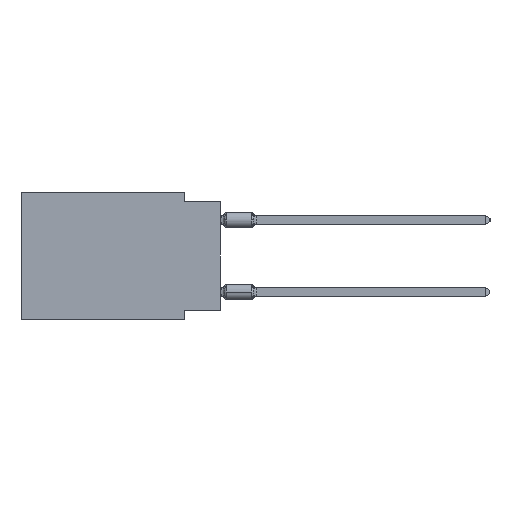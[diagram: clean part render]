
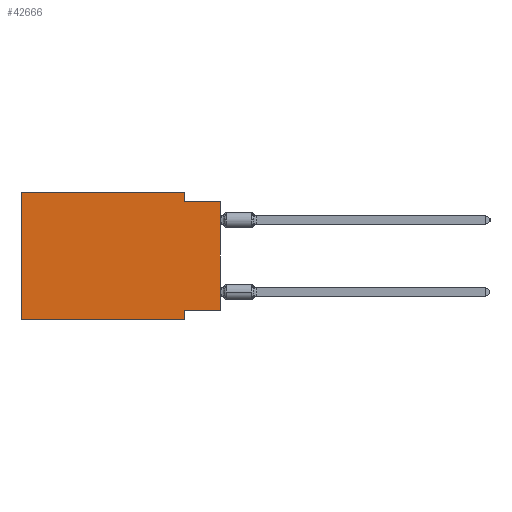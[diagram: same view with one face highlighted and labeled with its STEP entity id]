
A CAD part, left-side view. The second image highlights one B-rep face of the part: STEP entity #42666.
In plain terms, the highlighted planar face has unit normal (-1, 0, 0).
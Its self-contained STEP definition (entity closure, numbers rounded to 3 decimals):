
#12 = DIRECTION ( 'NONE',  ( 0., 0., -1. ) ) ;
#347 = LINE ( 'NONE', #47670, #58235 ) ;
#3822 = ORIENTED_EDGE ( 'NONE', *, *, #8270, .F. ) ;
#6979 = LINE ( 'NONE', #64171, #62223 ) ;
#8270 = EDGE_CURVE ( 'NONE', #39249, #8826, #15601, .T. ) ;
#8386 = DIRECTION ( 'NONE',  ( 0., 0., -1. ) ) ;
#8826 = VERTEX_POINT ( 'NONE', #8982 ) ;
#8982 = CARTESIAN_POINT ( 'NONE',  ( 0., 2.54, 0. ) ) ;
#9787 = CARTESIAN_POINT ( 'NONE',  ( 0., 13.97, -8.89 ) ) ;
#10345 = VECTOR ( 'NONE', #23052, 1000. ) ;
#11784 = VERTEX_POINT ( 'NONE', #9787 ) ;
#13386 = CARTESIAN_POINT ( 'NONE',  ( 0., 0., -8.255 ) ) ;
#14992 = VECTOR ( 'NONE', #37875, 1000. ) ;
#15601 = LINE ( 'NONE', #37076, #10345 ) ;
#16454 = ORIENTED_EDGE ( 'NONE', *, *, #60816, .F. ) ;
#16537 = VERTEX_POINT ( 'NONE', #35036 ) ;
#18549 = CARTESIAN_POINT ( 'NONE',  ( 0., 13.97, -8.89 ) ) ;
#19288 = VECTOR ( 'NONE', #8386, 1000. ) ;
#20458 = ORIENTED_EDGE ( 'NONE', *, *, #52609, .F. ) ;
#21287 = ORIENTED_EDGE ( 'NONE', *, *, #45430, .F. ) ;
#21473 = CARTESIAN_POINT ( 'NONE',  ( 0., 13.97, 0. ) ) ;
#21499 = VERTEX_POINT ( 'NONE', #23195 ) ;
#22657 = DIRECTION ( 'NONE',  ( 0., -1., 0. ) ) ;
#23052 = DIRECTION ( 'NONE',  ( 0., -1., 0. ) ) ;
#23195 = CARTESIAN_POINT ( 'NONE',  ( 0., 0., -0.635 ) ) ;
#23484 = VECTOR ( 'NONE', #48010, 1000. ) ;
#26127 = PLANE ( 'NONE',  #55648 ) ;
#27966 = LINE ( 'NONE', #47383, #14992 ) ;
#29496 = CARTESIAN_POINT ( 'NONE',  ( 0., 2.54, -8.89 ) ) ;
#30694 = CARTESIAN_POINT ( 'NONE',  ( 0., 2.54, -8.255 ) ) ;
#32631 = LINE ( 'NONE', #18549, #38567 ) ;
#35036 = CARTESIAN_POINT ( 'NONE',  ( 0., 2.54, -8.89 ) ) ;
#35334 = FACE_OUTER_BOUND ( 'NONE', #65254, .T. ) ;
#36827 = LINE ( 'NONE', #21473, #23484 ) ;
#36935 = CARTESIAN_POINT ( 'NONE',  ( 0., 2.54, -0.635 ) ) ;
#37076 = CARTESIAN_POINT ( 'NONE',  ( 0., 13.97, 0. ) ) ;
#37233 = ORIENTED_EDGE ( 'NONE', *, *, #44476, .T. ) ;
#37875 = DIRECTION ( 'NONE',  ( 0., 0., 1. ) ) ;
#38225 = VERTEX_POINT ( 'NONE', #30694 ) ;
#38567 = VECTOR ( 'NONE', #65507, 1000. ) ;
#39249 = VERTEX_POINT ( 'NONE', #64773 ) ;
#40984 = VERTEX_POINT ( 'NONE', #36935 ) ;
#42666 = ADVANCED_FACE ( 'NONE', ( #35334 ), #26127, .F. ) ;
#44476 = EDGE_CURVE ( 'NONE', #11784, #16537, #32631, .T. ) ;
#45430 = EDGE_CURVE ( 'NONE', #8826, #40984, #347, .T. ) ;
#45903 = LINE ( 'NONE', #50675, #51646 ) ;
#46339 = ORIENTED_EDGE ( 'NONE', *, *, #50164, .F. ) ;
#47383 = CARTESIAN_POINT ( 'NONE',  ( 0., 0., 0. ) ) ;
#47670 = CARTESIAN_POINT ( 'NONE',  ( 0., 2.54, 0. ) ) ;
#48010 = DIRECTION ( 'NONE',  ( 0., 0., 1. ) ) ;
#50164 = EDGE_CURVE ( 'NONE', #56490, #38225, #45903, .T. ) ;
#50652 = CARTESIAN_POINT ( 'NONE',  ( 0., 13.97, 0. ) ) ;
#50675 = CARTESIAN_POINT ( 'NONE',  ( 0., 0., -8.255 ) ) ;
#50937 = LINE ( 'NONE', #29496, #19288 ) ;
#51646 = VECTOR ( 'NONE', #66642, 1000. ) ;
#52609 = EDGE_CURVE ( 'NONE', #38225, #16537, #50937, .T. ) ;
#55648 = AXIS2_PLACEMENT_3D ( 'NONE', #50652, #66965, #56757 ) ;
#55704 = ORIENTED_EDGE ( 'NONE', *, *, #60452, .F. ) ;
#56490 = VERTEX_POINT ( 'NONE', #13386 ) ;
#56757 = DIRECTION ( 'NONE',  ( 0., 0., -1. ) ) ;
#58235 = VECTOR ( 'NONE', #12, 1000. ) ;
#60452 = EDGE_CURVE ( 'NONE', #11784, #39249, #36827, .T. ) ;
#60816 = EDGE_CURVE ( 'NONE', #40984, #21499, #6979, .T. ) ;
#62223 = VECTOR ( 'NONE', #22657, 1000. ) ;
#64171 = CARTESIAN_POINT ( 'NONE',  ( 0., 0., -0.635 ) ) ;
#64773 = CARTESIAN_POINT ( 'NONE',  ( 0., 13.97, 0. ) ) ;
#65013 = ORIENTED_EDGE ( 'NONE', *, *, #66057, .T. ) ;
#65254 = EDGE_LOOP ( 'NONE', ( #65013, #16454, #21287, #3822, #55704, #37233, #20458, #46339 ) ) ;
#65507 = DIRECTION ( 'NONE',  ( 0., -1., 0. ) ) ;
#66057 = EDGE_CURVE ( 'NONE', #56490, #21499, #27966, .T. ) ;
#66642 = DIRECTION ( 'NONE',  ( 0., 1., 0. ) ) ;
#66965 = DIRECTION ( 'NONE',  ( 1., 0., 0. ) ) ;
